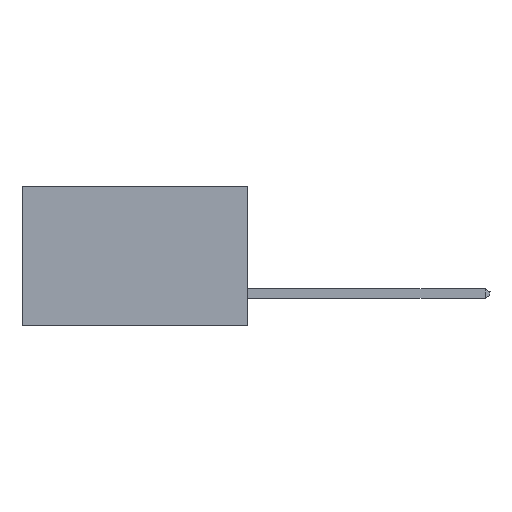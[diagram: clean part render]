
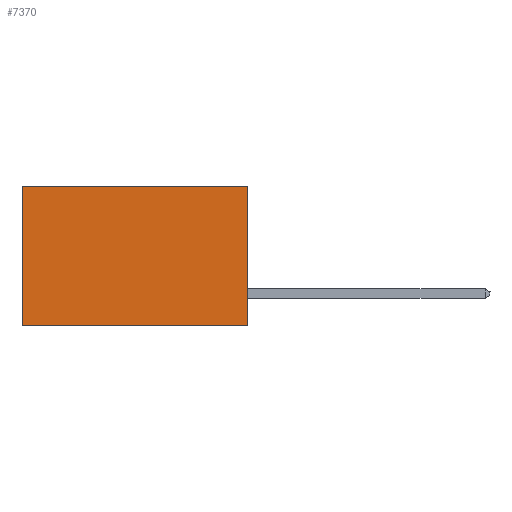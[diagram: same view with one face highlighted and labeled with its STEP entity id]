
A CAD part, left-side view. The second image highlights one B-rep face of the part: STEP entity #7370.
In plain terms, the highlighted planar face has unit normal (-1, 0, 0).
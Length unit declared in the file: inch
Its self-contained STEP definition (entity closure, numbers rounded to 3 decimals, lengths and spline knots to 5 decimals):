
#11 = ORIENTED_EDGE ( 'NONE', *, *, #5896, .T. ) ;
#448 = CARTESIAN_POINT ( 'NONE',  ( 0.2615, 0., -0.37 ) ) ;
#580 = CARTESIAN_POINT ( 'NONE',  ( 0.2615, 0., 0. ) ) ;
#1578 = EDGE_CURVE ( 'NONE', #4526, #12222, #10737, .T. ) ;
#1815 = LINE ( 'NONE', #3800, #3895 ) ;
#2112 = DIRECTION ( 'NONE',  ( 1., 0., 0. ) ) ;
#3155 = EDGE_CURVE ( 'NONE', #12222, #3633, #1815, .T. ) ;
#3633 = VERTEX_POINT ( 'NONE', #6863 ) ;
#3800 = CARTESIAN_POINT ( 'NONE',  ( 0.2615, 0., -0.37 ) ) ;
#3895 = VECTOR ( 'NONE', #8106, 39.37008 ) ;
#4167 = CARTESIAN_POINT ( 'NONE',  ( 0.2615, 0., -0.37 ) ) ;
#4526 = VERTEX_POINT ( 'NONE', #11946 ) ;
#4603 = DIRECTION ( 'NONE',  ( 0., 0., -1. ) ) ;
#5401 = ORIENTED_EDGE ( 'NONE', *, *, #1578, .F. ) ;
#5678 = LINE ( 'NONE', #580, #13119 ) ;
#5743 = EDGE_CURVE ( 'NONE', #12777, #3633, #6137, .T. ) ;
#5896 = EDGE_CURVE ( 'NONE', #4526, #12777, #5678, .T. ) ;
#6137 = LINE ( 'NONE', #6621, #7728 ) ;
#6305 = ORIENTED_EDGE ( 'NONE', *, *, #3155, .F. ) ;
#6621 = CARTESIAN_POINT ( 'NONE',  ( 0.2615, 0.6, -0.37 ) ) ;
#6863 = CARTESIAN_POINT ( 'NONE',  ( 0.2615, 0.6, -0.37 ) ) ;
#7370 = ADVANCED_FACE ( 'NONE', ( #12512 ), #12376, .F. ) ;
#7544 = VECTOR ( 'NONE', #4603, 39.37008 ) ;
#7728 = VECTOR ( 'NONE', #10651, 39.37008 ) ;
#8106 = DIRECTION ( 'NONE',  ( 0., 1., 0. ) ) ;
#8121 = CARTESIAN_POINT ( 'NONE',  ( 0.2615, 0.6, 0. ) ) ;
#8983 = DIRECTION ( 'NONE',  ( 0., 1., 0. ) ) ;
#10518 = AXIS2_PLACEMENT_3D ( 'NONE', #4167, #2112, #12633 ) ;
#10651 = DIRECTION ( 'NONE',  ( 0., 0., -1. ) ) ;
#10737 = LINE ( 'NONE', #448, #7544 ) ;
#11403 = CARTESIAN_POINT ( 'NONE',  ( 0.2615, 0., -0.37 ) ) ;
#11946 = CARTESIAN_POINT ( 'NONE',  ( 0.2615, 0., 0. ) ) ;
#12023 = ORIENTED_EDGE ( 'NONE', *, *, #5743, .T. ) ;
#12222 = VERTEX_POINT ( 'NONE', #11403 ) ;
#12376 = PLANE ( 'NONE',  #10518 ) ;
#12512 = FACE_OUTER_BOUND ( 'NONE', #13142, .T. ) ;
#12633 = DIRECTION ( 'NONE',  ( 0., 0., -1. ) ) ;
#12777 = VERTEX_POINT ( 'NONE', #8121 ) ;
#13119 = VECTOR ( 'NONE', #8983, 39.37008 ) ;
#13142 = EDGE_LOOP ( 'NONE', ( #12023, #6305, #5401, #11 ) ) ;
